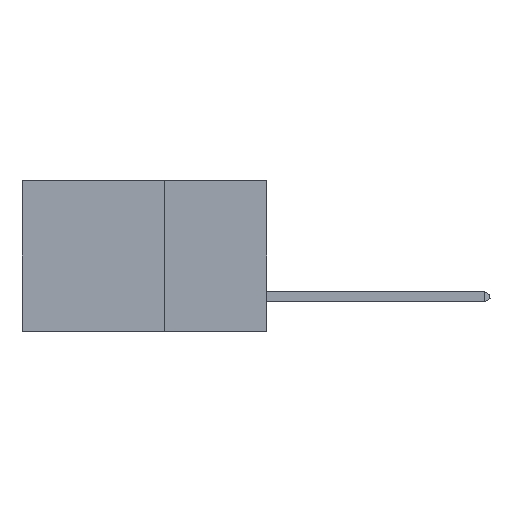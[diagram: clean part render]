
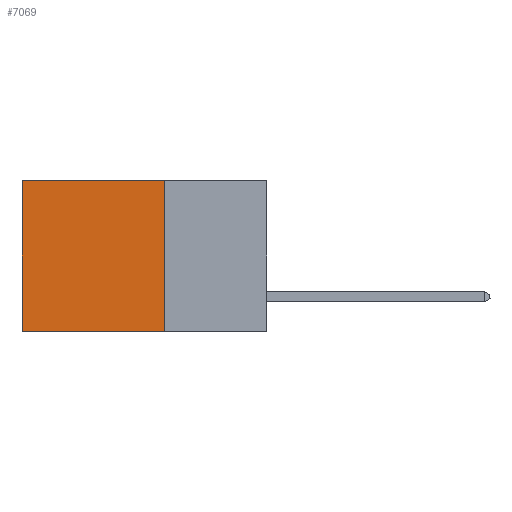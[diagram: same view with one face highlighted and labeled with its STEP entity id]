
A CAD part, left-side view. The second image highlights one B-rep face of the part: STEP entity #7069.
In plain terms, the highlighted planar face has unit normal (-1, 0, 0).
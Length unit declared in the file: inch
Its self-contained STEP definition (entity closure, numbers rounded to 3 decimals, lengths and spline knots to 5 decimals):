
#572 = ORIENTED_EDGE ( 'NONE', *, *, #37968, .F. ) ;
#2439 = LINE ( 'NONE', #10915, #10085 ) ;
#2688 = VERTEX_POINT ( 'NONE', #3299 ) ;
#3299 = CARTESIAN_POINT ( 'NONE',  ( 0.2875, 0.25, 0. ) ) ;
#4398 = VERTEX_POINT ( 'NONE', #39508 ) ;
#4826 = DIRECTION ( 'NONE',  ( 0., 1., 0. ) ) ;
#5038 = LINE ( 'NONE', #24060, #6068 ) ;
#5080 = LINE ( 'NONE', #27584, #38621 ) ;
#6068 = VECTOR ( 'NONE', #14048, 39.37008 ) ;
#7069 = ADVANCED_FACE ( 'NONE', ( #9379 ), #33776, .F. ) ;
#9379 = FACE_OUTER_BOUND ( 'NONE', #39869, .T. ) ;
#10085 = VECTOR ( 'NONE', #4826, 39.37008 ) ;
#10605 = ORIENTED_EDGE ( 'NONE', *, *, #33729, .F. ) ;
#10638 = ORIENTED_EDGE ( 'NONE', *, *, #32610, .T. ) ;
#10915 = CARTESIAN_POINT ( 'NONE',  ( 0.2875, 0.25, -0.37 ) ) ;
#14048 = DIRECTION ( 'NONE',  ( 0., 0., -1. ) ) ;
#18661 = DIRECTION ( 'NONE',  ( 0., 1., 0. ) ) ;
#23051 = CARTESIAN_POINT ( 'NONE',  ( 0.2875, 0.25, 0. ) ) ;
#24060 = CARTESIAN_POINT ( 'NONE',  ( 0.2875, 0.6, 0. ) ) ;
#26440 = DIRECTION ( 'NONE',  ( 0., 0., -1. ) ) ;
#26512 = LINE ( 'NONE', #23051, #32632 ) ;
#27584 = CARTESIAN_POINT ( 'NONE',  ( 0.2875, 0.25, 0. ) ) ;
#32610 = EDGE_CURVE ( 'NONE', #2688, #4398, #5080, .T. ) ;
#32632 = VECTOR ( 'NONE', #26440, 39.37008 ) ;
#33729 = EDGE_CURVE ( 'NONE', #41086, #41032, #2439, .T. ) ;
#33776 = PLANE ( 'NONE',  #33884 ) ;
#33826 = DIRECTION ( 'NONE',  ( 0., 0., -1. ) ) ;
#33884 = AXIS2_PLACEMENT_3D ( 'NONE', #41427, #35826, #33826 ) ;
#35826 = DIRECTION ( 'NONE',  ( 1., 0., 0. ) ) ;
#35987 = CARTESIAN_POINT ( 'NONE',  ( 0.2875, 0.6, -0.37 ) ) ;
#37968 = EDGE_CURVE ( 'NONE', #2688, #41086, #26512, .T. ) ;
#38609 = EDGE_CURVE ( 'NONE', #4398, #41032, #5038, .T. ) ;
#38621 = VECTOR ( 'NONE', #18661, 39.37008 ) ;
#39378 = CARTESIAN_POINT ( 'NONE',  ( 0.2875, 0.25, -0.37 ) ) ;
#39508 = CARTESIAN_POINT ( 'NONE',  ( 0.2875, 0.6, 0. ) ) ;
#39869 = EDGE_LOOP ( 'NONE', ( #41239, #10605, #572, #10638 ) ) ;
#41032 = VERTEX_POINT ( 'NONE', #35987 ) ;
#41086 = VERTEX_POINT ( 'NONE', #39378 ) ;
#41239 = ORIENTED_EDGE ( 'NONE', *, *, #38609, .T. ) ;
#41427 = CARTESIAN_POINT ( 'NONE',  ( 0.2875, 0.25, 0. ) ) ;
